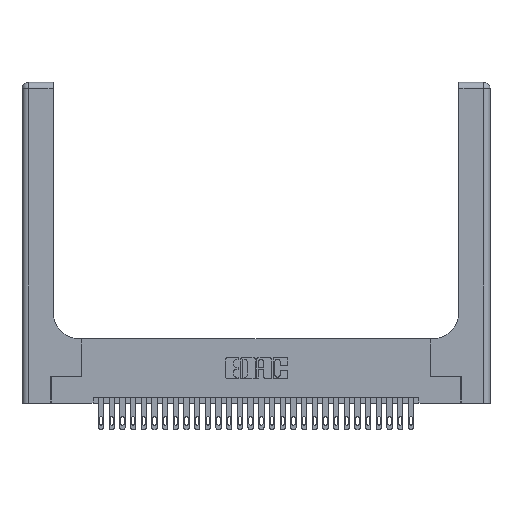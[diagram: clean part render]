
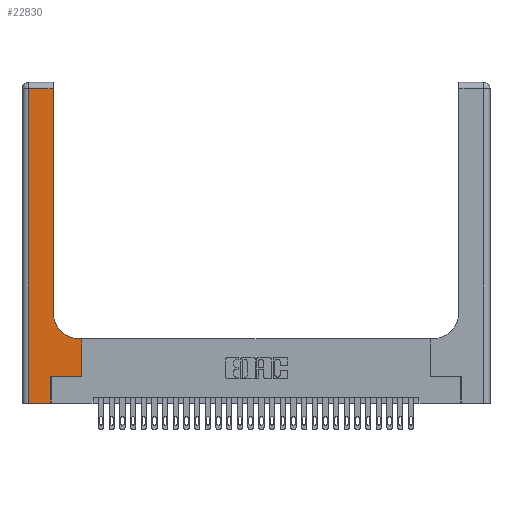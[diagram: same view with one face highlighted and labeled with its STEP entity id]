
A CAD part, top view. The second image highlights one B-rep face of the part: STEP entity #22830.
In plain terms, the highlighted planar face has unit normal (0, 0, 1).
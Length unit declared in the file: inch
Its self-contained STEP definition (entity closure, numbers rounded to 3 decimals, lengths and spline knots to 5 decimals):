
#1006 = VERTEX_POINT ( 'NONE', #22087 ) ;
#1551 = CARTESIAN_POINT ( 'NONE',  ( 0.269, 0., 0.37 ) ) ;
#2035 = VECTOR ( 'NONE', #27474, 39.37008 ) ;
#2103 = EDGE_CURVE ( 'NONE', #23528, #6735, #22431, .T. ) ;
#3157 = VERTEX_POINT ( 'NONE', #7451 ) ;
#3561 = LINE ( 'NONE', #24223, #7564 ) ;
#3672 = VECTOR ( 'NONE', #22104, 39.37008 ) ;
#3906 = DIRECTION ( 'NONE',  ( -1., 0., 0. ) ) ;
#3970 = CARTESIAN_POINT ( 'NONE',  ( 0., 2.94, 0.37 ) ) ;
#4403 = LINE ( 'NONE', #25675, #28547 ) ;
#4883 = ORIENTED_EDGE ( 'NONE', *, *, #29271, .T. ) ;
#4898 = ORIENTED_EDGE ( 'NONE', *, *, #24460, .T. ) ;
#5108 = VECTOR ( 'NONE', #13035, 39.37008 ) ;
#5124 = DIRECTION ( 'NONE',  ( 0., 1., 0. ) ) ;
#5828 = DIRECTION ( 'NONE',  ( 0., 0., -1. ) ) ;
#6142 = PLANE ( 'NONE',  #9826 ) ;
#6523 = EDGE_CURVE ( 'NONE', #28652, #21595, #27913, .T. ) ;
#6567 = ORIENTED_EDGE ( 'NONE', *, *, #2103, .T. ) ;
#6735 = VERTEX_POINT ( 'NONE', #7650 ) ;
#7451 = CARTESIAN_POINT ( 'NONE',  ( 0.06, 2.94, 0.37 ) ) ;
#7452 = VECTOR ( 'NONE', #13585, 39.37008 ) ;
#7564 = VECTOR ( 'NONE', #5124, 39.37008 ) ;
#7650 = CARTESIAN_POINT ( 'NONE',  ( 0.269, 0.25, 0.37 ) ) ;
#7948 = EDGE_CURVE ( 'NONE', #13412, #28652, #14569, .T. ) ;
#8011 = VECTOR ( 'NONE', #21496, 39.37008 ) ;
#8060 = VERTEX_POINT ( 'NONE', #28392 ) ;
#8916 = ORIENTED_EDGE ( 'NONE', *, *, #15651, .T. ) ;
#9595 = CARTESIAN_POINT ( 'NONE',  ( 0.06, 3., 0.37 ) ) ;
#9826 = AXIS2_PLACEMENT_3D ( 'NONE', #17637, #5828, #3906 ) ;
#10701 = ORIENTED_EDGE ( 'NONE', *, *, #13400, .T. ) ;
#11664 = CARTESIAN_POINT ( 'NONE',  ( 0.269, 0., 0.37 ) ) ;
#12093 = CARTESIAN_POINT ( 'NONE',  ( 0.2915, 2.94, 0.37 ) ) ;
#13035 = DIRECTION ( 'NONE',  ( -1., 0., 0. ) ) ;
#13400 = EDGE_CURVE ( 'NONE', #3157, #8060, #24431, .T. ) ;
#13412 = VERTEX_POINT ( 'NONE', #26361 ) ;
#13585 = DIRECTION ( 'NONE',  ( 0., 1., 0. ) ) ;
#14190 = EDGE_LOOP ( 'NONE', ( #4883, #8916, #10701, #17619, #6567, #28422, #4898, #21285, #25189 ) ) ;
#14382 = CARTESIAN_POINT ( 'NONE',  ( 0.5415, 0.6, 0.37 ) ) ;
#14569 = LINE ( 'NONE', #19773, #5108 ) ;
#15651 = EDGE_CURVE ( 'NONE', #15830, #3157, #18810, .T. ) ;
#15830 = VERTEX_POINT ( 'NONE', #12093 ) ;
#16144 = DIRECTION ( 'NONE',  ( 1., 0., 0. ) ) ;
#17001 = CARTESIAN_POINT ( 'NONE',  ( 0.2915, 3., 0.37 ) ) ;
#17619 = ORIENTED_EDGE ( 'NONE', *, *, #22075, .T. ) ;
#17637 = CARTESIAN_POINT ( 'NONE',  ( 0., 3., 0.37 ) ) ;
#18350 = DIRECTION ( 'NONE',  ( 0., 0., -1. ) ) ;
#18810 = LINE ( 'NONE', #3970, #2035 ) ;
#19657 = VECTOR ( 'NONE', #23979, 39.37008 ) ;
#19761 = CARTESIAN_POINT ( 'NONE',  ( 0., 0., 0.37 ) ) ;
#19773 = CARTESIAN_POINT ( 'NONE',  ( 0.2915, 0.6, 0.37 ) ) ;
#21175 = AXIS2_PLACEMENT_3D ( 'NONE', #30275, #18350, #22791 ) ;
#21285 = ORIENTED_EDGE ( 'NONE', *, *, #7948, .T. ) ;
#21496 = DIRECTION ( 'NONE',  ( 0., 1., 0. ) ) ;
#21595 = VERTEX_POINT ( 'NONE', #29535 ) ;
#22075 = EDGE_CURVE ( 'NONE', #8060, #23528, #30034, .T. ) ;
#22087 = CARTESIAN_POINT ( 'NONE',  ( 0.5585, 0.25, 0.37 ) ) ;
#22104 = DIRECTION ( 'NONE',  ( 1., 0., 0. ) ) ;
#22293 = EDGE_CURVE ( 'NONE', #6735, #1006, #4403, .T. ) ;
#22431 = LINE ( 'NONE', #11664, #7452 ) ;
#22791 = DIRECTION ( 'NONE',  ( 1., 0., 0. ) ) ;
#22830 = ADVANCED_FACE ( 'NONE', ( #24074 ), #6142, .F. ) ;
#23528 = VERTEX_POINT ( 'NONE', #1551 ) ;
#23979 = DIRECTION ( 'NONE',  ( 0., -1., 0. ) ) ;
#24074 = FACE_OUTER_BOUND ( 'NONE', #14190, .T. ) ;
#24223 = CARTESIAN_POINT ( 'NONE',  ( 0.5585, 0.25, 0.37 ) ) ;
#24431 = LINE ( 'NONE', #9595, #19657 ) ;
#24460 = EDGE_CURVE ( 'NONE', #1006, #13412, #3561, .T. ) ;
#25189 = ORIENTED_EDGE ( 'NONE', *, *, #6523, .T. ) ;
#25675 = CARTESIAN_POINT ( 'NONE',  ( 0.269, 0.25, 0.37 ) ) ;
#26361 = CARTESIAN_POINT ( 'NONE',  ( 0.5585, 0.6, 0.37 ) ) ;
#27474 = DIRECTION ( 'NONE',  ( -1., 0., 0. ) ) ;
#27913 = CIRCLE ( 'NONE', #21175, 0.25 ) ;
#28392 = CARTESIAN_POINT ( 'NONE',  ( 0.06, 0., 0.37 ) ) ;
#28422 = ORIENTED_EDGE ( 'NONE', *, *, #22293, .T. ) ;
#28547 = VECTOR ( 'NONE', #16144, 39.37008 ) ;
#28652 = VERTEX_POINT ( 'NONE', #14382 ) ;
#28867 = LINE ( 'NONE', #17001, #8011 ) ;
#29271 = EDGE_CURVE ( 'NONE', #21595, #15830, #28867, .T. ) ;
#29535 = CARTESIAN_POINT ( 'NONE',  ( 0.2915, 0.85, 0.37 ) ) ;
#30034 = LINE ( 'NONE', #19761, #3672 ) ;
#30275 = CARTESIAN_POINT ( 'NONE',  ( 0.5415, 0.85, 0.37 ) ) ;
